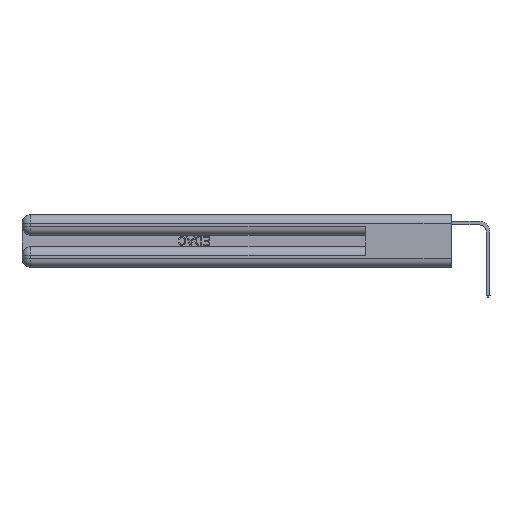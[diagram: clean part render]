
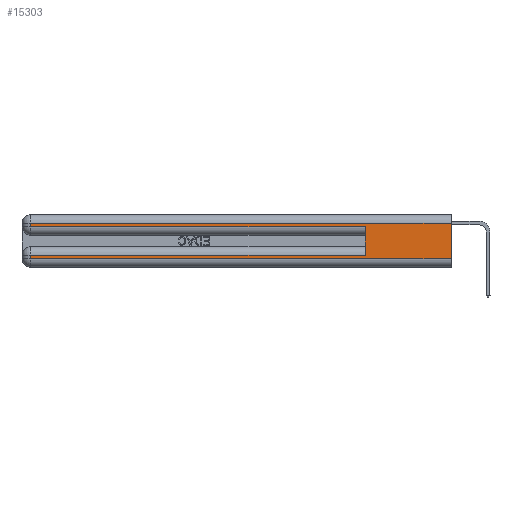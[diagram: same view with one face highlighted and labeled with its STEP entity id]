
A CAD part, left-side view. The second image highlights one B-rep face of the part: STEP entity #15303.
In plain terms, the highlighted planar face has unit normal (-1, 0, 0).
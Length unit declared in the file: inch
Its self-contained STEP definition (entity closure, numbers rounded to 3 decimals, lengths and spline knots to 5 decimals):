
#230 = LINE ( 'NONE', #7785, #8663 ) ;
#913 = CARTESIAN_POINT ( 'NONE',  ( 0., 0., 0.285 ) ) ;
#1397 = EDGE_CURVE ( 'NONE', #17305, #19922, #230, .T. ) ;
#1693 = CARTESIAN_POINT ( 'NONE',  ( 0., 0.6, 0.285 ) ) ;
#2468 = CARTESIAN_POINT ( 'NONE',  ( 0., 2.94, 0.06 ) ) ;
#2627 = ORIENTED_EDGE ( 'NONE', *, *, #29618, .T. ) ;
#2731 = DIRECTION ( 'NONE',  ( 0., 0., -1. ) ) ;
#2906 = VECTOR ( 'NONE', #8297, 39.37008 ) ;
#3286 = ORIENTED_EDGE ( 'NONE', *, *, #8143, .F. ) ;
#3619 = EDGE_CURVE ( 'NONE', #9631, #18701, #20728, .T. ) ;
#4408 = EDGE_CURVE ( 'NONE', #14975, #17305, #9747, .T. ) ;
#4433 = CARTESIAN_POINT ( 'NONE',  ( 0., 0.6, 0.145 ) ) ;
#4830 = VECTOR ( 'NONE', #14681, 39.37008 ) ;
#5663 = CARTESIAN_POINT ( 'NONE',  ( 0., 0., 0.31 ) ) ;
#6971 = VECTOR ( 'NONE', #21268, 39.37008 ) ;
#7471 = VERTEX_POINT ( 'NONE', #1693 ) ;
#7785 = CARTESIAN_POINT ( 'NONE',  ( 0., 2.94, 0.37 ) ) ;
#8143 = EDGE_CURVE ( 'NONE', #24833, #7471, #14173, .T. ) ;
#8297 = DIRECTION ( 'NONE',  ( 0., -1., 0. ) ) ;
#8663 = VECTOR ( 'NONE', #2731, 39.37008 ) ;
#8971 = VECTOR ( 'NONE', #28513, 39.37008 ) ;
#9631 = VERTEX_POINT ( 'NONE', #2468 ) ;
#9747 = LINE ( 'NONE', #30630, #15277 ) ;
#10483 = LINE ( 'NONE', #10983, #6971 ) ;
#10810 = LINE ( 'NONE', #913, #8971 ) ;
#10983 = CARTESIAN_POINT ( 'NONE',  ( 0., 0., 0.37 ) ) ;
#11486 = VECTOR ( 'NONE', #22133, 39.37008 ) ;
#13577 = AXIS2_PLACEMENT_3D ( 'NONE', #23623, #28315, #28496 ) ;
#14173 = LINE ( 'NONE', #4433, #21951 ) ;
#14681 = DIRECTION ( 'NONE',  ( 0., 0., -1. ) ) ;
#14975 = VERTEX_POINT ( 'NONE', #5663 ) ;
#15277 = VECTOR ( 'NONE', #30288, 39.37008 ) ;
#15303 = ADVANCED_FACE ( 'NONE', ( #28664 ), #31202, .F. ) ;
#16210 = EDGE_CURVE ( 'NONE', #24833, #26088, #24137, .T. ) ;
#17305 = VERTEX_POINT ( 'NONE', #19319 ) ;
#17766 = EDGE_LOOP ( 'NONE', ( #23409, #17869, #24608, #2627, #3286, #31783, #28134, #32012 ) ) ;
#17869 = ORIENTED_EDGE ( 'NONE', *, *, #4408, .T. ) ;
#18701 = VERTEX_POINT ( 'NONE', #20331 ) ;
#19319 = CARTESIAN_POINT ( 'NONE',  ( 0., 2.94, 0.31 ) ) ;
#19922 = VERTEX_POINT ( 'NONE', #22772 ) ;
#20331 = CARTESIAN_POINT ( 'NONE',  ( 0., 0., 0.06 ) ) ;
#20557 = LINE ( 'NONE', #30164, #4830 ) ;
#20728 = LINE ( 'NONE', #23433, #2906 ) ;
#20752 = CARTESIAN_POINT ( 'NONE',  ( 0., 0.6, 0.085 ) ) ;
#21268 = DIRECTION ( 'NONE',  ( 0., 0., -1. ) ) ;
#21476 = CARTESIAN_POINT ( 'NONE',  ( 0., 2.94, 0.085 ) ) ;
#21951 = VECTOR ( 'NONE', #22422, 39.37008 ) ;
#22133 = DIRECTION ( 'NONE',  ( 0., 1., 0. ) ) ;
#22422 = DIRECTION ( 'NONE',  ( 0., 0., 1. ) ) ;
#22772 = CARTESIAN_POINT ( 'NONE',  ( 0., 2.94, 0.285 ) ) ;
#23409 = ORIENTED_EDGE ( 'NONE', *, *, #30796, .F. ) ;
#23433 = CARTESIAN_POINT ( 'NONE',  ( 0., 0., 0.06 ) ) ;
#23623 = CARTESIAN_POINT ( 'NONE',  ( 0., 0., 0.37 ) ) ;
#24137 = LINE ( 'NONE', #24306, #11486 ) ;
#24306 = CARTESIAN_POINT ( 'NONE',  ( 0., 0., 0.085 ) ) ;
#24608 = ORIENTED_EDGE ( 'NONE', *, *, #1397, .T. ) ;
#24833 = VERTEX_POINT ( 'NONE', #20752 ) ;
#26088 = VERTEX_POINT ( 'NONE', #21476 ) ;
#28134 = ORIENTED_EDGE ( 'NONE', *, *, #31099, .T. ) ;
#28315 = DIRECTION ( 'NONE',  ( 1., 0., 0. ) ) ;
#28496 = DIRECTION ( 'NONE',  ( 0., 0., -1. ) ) ;
#28513 = DIRECTION ( 'NONE',  ( 0., -1., 0. ) ) ;
#28664 = FACE_OUTER_BOUND ( 'NONE', #17766, .T. ) ;
#29618 = EDGE_CURVE ( 'NONE', #19922, #7471, #10810, .T. ) ;
#30164 = CARTESIAN_POINT ( 'NONE',  ( 0., 2.94, 0.37 ) ) ;
#30288 = DIRECTION ( 'NONE',  ( 0., 1., 0. ) ) ;
#30630 = CARTESIAN_POINT ( 'NONE',  ( 0., 0., 0.31 ) ) ;
#30796 = EDGE_CURVE ( 'NONE', #14975, #18701, #10483, .T. ) ;
#31099 = EDGE_CURVE ( 'NONE', #26088, #9631, #20557, .T. ) ;
#31202 = PLANE ( 'NONE',  #13577 ) ;
#31783 = ORIENTED_EDGE ( 'NONE', *, *, #16210, .T. ) ;
#32012 = ORIENTED_EDGE ( 'NONE', *, *, #3619, .T. ) ;
